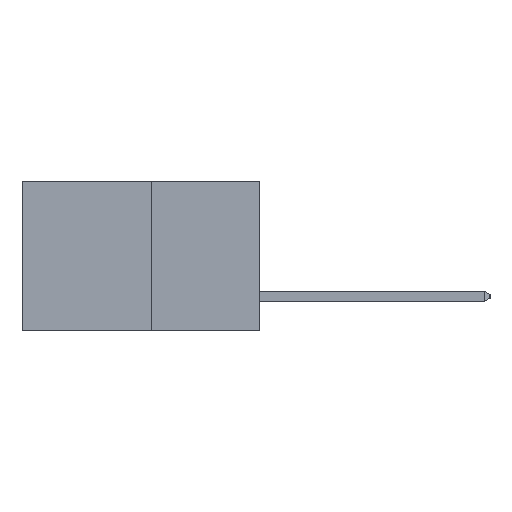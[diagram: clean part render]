
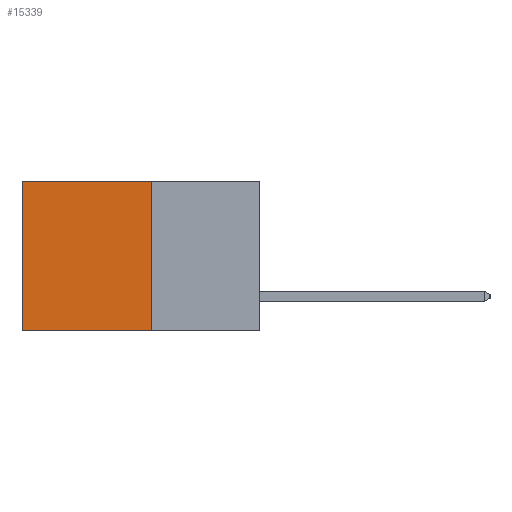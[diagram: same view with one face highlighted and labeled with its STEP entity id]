
A CAD part, left-side view. The second image highlights one B-rep face of the part: STEP entity #15339.
In plain terms, the highlighted planar face has unit normal (-1, 0, 0).
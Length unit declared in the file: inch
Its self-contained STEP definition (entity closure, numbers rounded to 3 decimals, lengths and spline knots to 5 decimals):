
#160 = CARTESIAN_POINT ( 'NONE',  ( 0.277, 0.27, 0. ) ) ;
#176 = LINE ( 'NONE', #11839, #16033 ) ;
#1306 = EDGE_CURVE ( 'NONE', #17044, #10628, #4627, .T. ) ;
#1863 = CARTESIAN_POINT ( 'NONE',  ( 0.277, 0.59, -0.37 ) ) ;
#1990 = LINE ( 'NONE', #11701, #5595 ) ;
#2707 = CARTESIAN_POINT ( 'NONE',  ( 0.277, 0.59, -0.37 ) ) ;
#2725 = CARTESIAN_POINT ( 'NONE',  ( 0.277, 0.27, 0. ) ) ;
#3386 = DIRECTION ( 'NONE',  ( 0., 0., -1. ) ) ;
#4627 = LINE ( 'NONE', #2725, #12866 ) ;
#4732 = FACE_OUTER_BOUND ( 'NONE', #16523, .T. ) ;
#4837 = VERTEX_POINT ( 'NONE', #18088 ) ;
#5595 = VECTOR ( 'NONE', #7103, 39.37008 ) ;
#6123 = EDGE_CURVE ( 'NONE', #4837, #10000, #176, .T. ) ;
#7103 = DIRECTION ( 'NONE',  ( 0., 0., -1. ) ) ;
#8203 = DIRECTION ( 'NONE',  ( 0., 1., 0. ) ) ;
#8412 = DIRECTION ( 'NONE',  ( 1., 0., 0. ) ) ;
#10000 = VERTEX_POINT ( 'NONE', #2707 ) ;
#10116 = AXIS2_PLACEMENT_3D ( 'NONE', #16069, #8412, #19056 ) ;
#10269 = EDGE_CURVE ( 'NONE', #10628, #10000, #13384, .T. ) ;
#10628 = VERTEX_POINT ( 'NONE', #11827 ) ;
#11448 = PLANE ( 'NONE',  #10116 ) ;
#11467 = ORIENTED_EDGE ( 'NONE', *, *, #18187, .F. ) ;
#11701 = CARTESIAN_POINT ( 'NONE',  ( 0.277, 0.27, -0.37 ) ) ;
#11827 = CARTESIAN_POINT ( 'NONE',  ( 0.277, 0.59, 0. ) ) ;
#11839 = CARTESIAN_POINT ( 'NONE',  ( 0.277, 0.27, -0.37 ) ) ;
#12316 = ORIENTED_EDGE ( 'NONE', *, *, #10269, .T. ) ;
#12866 = VECTOR ( 'NONE', #19255, 39.37008 ) ;
#13384 = LINE ( 'NONE', #1863, #16468 ) ;
#15339 = ADVANCED_FACE ( 'NONE', ( #4732 ), #11448, .F. ) ;
#16033 = VECTOR ( 'NONE', #8203, 39.37008 ) ;
#16069 = CARTESIAN_POINT ( 'NONE',  ( 0.277, 0.27, -0.37 ) ) ;
#16468 = VECTOR ( 'NONE', #3386, 39.37008 ) ;
#16523 = EDGE_LOOP ( 'NONE', ( #12316, #16921, #11467, #18443 ) ) ;
#16921 = ORIENTED_EDGE ( 'NONE', *, *, #6123, .F. ) ;
#17044 = VERTEX_POINT ( 'NONE', #160 ) ;
#18088 = CARTESIAN_POINT ( 'NONE',  ( 0.277, 0.27, -0.37 ) ) ;
#18187 = EDGE_CURVE ( 'NONE', #17044, #4837, #1990, .T. ) ;
#18443 = ORIENTED_EDGE ( 'NONE', *, *, #1306, .T. ) ;
#19056 = DIRECTION ( 'NONE',  ( 0., 0., -1. ) ) ;
#19255 = DIRECTION ( 'NONE',  ( 0., 1., 0. ) ) ;
